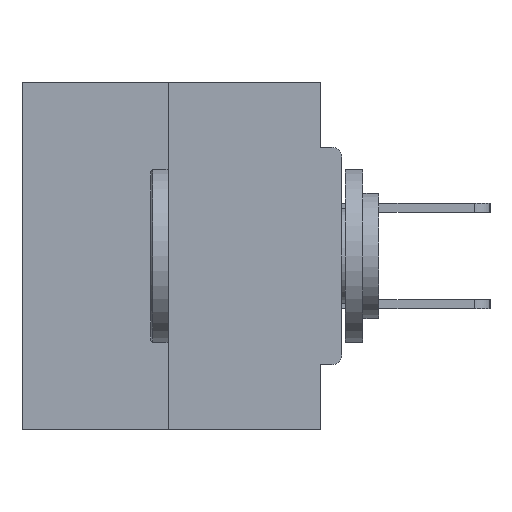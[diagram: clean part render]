
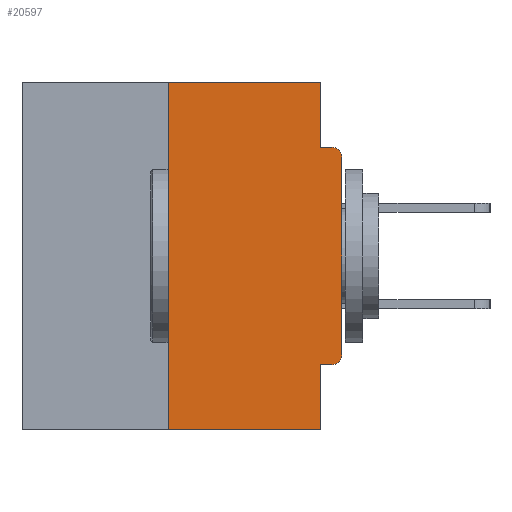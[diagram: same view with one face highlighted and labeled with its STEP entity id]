
A CAD part, left-side view. The second image highlights one B-rep face of the part: STEP entity #20597.
In plain terms, the highlighted planar face has unit normal (-1, 0, 0).
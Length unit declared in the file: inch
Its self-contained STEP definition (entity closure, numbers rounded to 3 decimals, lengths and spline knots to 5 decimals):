
#204 = LINE ( 'NONE', #33805, #28159 ) ;
#296 = ORIENTED_EDGE ( 'NONE', *, *, #18567, .F. ) ;
#996 = EDGE_CURVE ( 'NONE', #21128, #29124, #10618, .T. ) ;
#1128 = VECTOR ( 'NONE', #10268, 39.37008 ) ;
#2202 = VECTOR ( 'NONE', #10161, 39.37008 ) ;
#2663 = LINE ( 'NONE', #18475, #2202 ) ;
#3200 = EDGE_CURVE ( 'NONE', #29124, #3652, #204, .T. ) ;
#3307 = DIRECTION ( 'NONE',  ( 0., 0., -1. ) ) ;
#3652 = VERTEX_POINT ( 'NONE', #15938 ) ;
#4697 = CIRCLE ( 'NONE', #22567, 0.015 ) ;
#4855 = CARTESIAN_POINT ( 'NONE',  ( 0., 0.015, -0.4065 ) ) ;
#5638 = EDGE_CURVE ( 'NONE', #28299, #8201, #22615, .T. ) ;
#5758 = VECTOR ( 'NONE', #8541, 39.37008 ) ;
#5893 = EDGE_LOOP ( 'NONE', ( #32240, #16080, #33686, #9044, #9301, #25799, #20380, #15599, #296, #11956 ) ) ;
#5894 = CARTESIAN_POINT ( 'NONE',  ( 0., 0.25, -0.5 ) ) ;
#6037 = VECTOR ( 'NONE', #35505, 39.37008 ) ;
#6777 = PLANE ( 'NONE',  #25601 ) ;
#7136 = CARTESIAN_POINT ( 'NONE',  ( 0., 0.031, -0.5 ) ) ;
#7481 = VECTOR ( 'NONE', #20732, 39.37008 ) ;
#8165 = EDGE_CURVE ( 'NONE', #32360, #8201, #20238, .T. ) ;
#8201 = VERTEX_POINT ( 'NONE', #30403 ) ;
#8541 = DIRECTION ( 'NONE',  ( 0., -1., 0. ) ) ;
#9044 = ORIENTED_EDGE ( 'NONE', *, *, #8165, .F. ) ;
#9251 = CARTESIAN_POINT ( 'NONE',  ( 0., 0.015, -0.0935 ) ) ;
#9301 = ORIENTED_EDGE ( 'NONE', *, *, #29489, .F. ) ;
#10161 = DIRECTION ( 'NONE',  ( 0., 0., 1. ) ) ;
#10268 = DIRECTION ( 'NONE',  ( 0., 0., 1. ) ) ;
#10618 = LINE ( 'NONE', #22727, #5758 ) ;
#10646 = CARTESIAN_POINT ( 'NONE',  ( 0., 0.25, 0. ) ) ;
#10975 = CARTESIAN_POINT ( 'NONE',  ( 0., 0.031, -0.4065 ) ) ;
#11922 = AXIS2_PLACEMENT_3D ( 'NONE', #17479, #20595, #20360 ) ;
#11956 = ORIENTED_EDGE ( 'NONE', *, *, #3200, .F. ) ;
#12156 = VERTEX_POINT ( 'NONE', #12800 ) ;
#12324 = FACE_OUTER_BOUND ( 'NONE', #5893, .T. ) ;
#12800 = CARTESIAN_POINT ( 'NONE',  ( 0., 0., -0.1085 ) ) ;
#13571 = DIRECTION ( 'NONE',  ( 0., -1., 0. ) ) ;
#14453 = DIRECTION ( 'NONE',  ( -1., 0., 0. ) ) ;
#14869 = EDGE_CURVE ( 'NONE', #28299, #21128, #16214, .T. ) ;
#15599 = ORIENTED_EDGE ( 'NONE', *, *, #27118, .T. ) ;
#15611 = VERTEX_POINT ( 'NONE', #25151 ) ;
#15931 = VERTEX_POINT ( 'NONE', #4855 ) ;
#15938 = CARTESIAN_POINT ( 'NONE',  ( 0., 0.031, -0.0935 ) ) ;
#16080 = ORIENTED_EDGE ( 'NONE', *, *, #14869, .F. ) ;
#16214 = LINE ( 'NONE', #10646, #1128 ) ;
#17479 = CARTESIAN_POINT ( 'NONE',  ( 0., 0.015, -0.1085 ) ) ;
#18192 = EDGE_CURVE ( 'NONE', #15611, #12156, #2663, .T. ) ;
#18475 = CARTESIAN_POINT ( 'NONE',  ( 0., 0., 0. ) ) ;
#18567 = EDGE_CURVE ( 'NONE', #3652, #20509, #22167, .T. ) ;
#18777 = CARTESIAN_POINT ( 'NONE',  ( 0., 0.25, 0. ) ) ;
#19826 = DIRECTION ( 'NONE',  ( 0., 0., -1. ) ) ;
#20068 = DIRECTION ( 'NONE',  ( 0., 1., 0. ) ) ;
#20238 = LINE ( 'NONE', #7136, #6037 ) ;
#20360 = DIRECTION ( 'NONE',  ( 0., 0., -1. ) ) ;
#20380 = ORIENTED_EDGE ( 'NONE', *, *, #18192, .T. ) ;
#20509 = VERTEX_POINT ( 'NONE', #9251 ) ;
#20595 = DIRECTION ( 'NONE',  ( -1., 0., 0. ) ) ;
#20597 = ADVANCED_FACE ( 'NONE', ( #12324 ), #6777, .F. ) ;
#20599 = CARTESIAN_POINT ( 'NONE',  ( 0., 0.031, 0. ) ) ;
#20732 = DIRECTION ( 'NONE',  ( 0., -1., 0. ) ) ;
#21128 = VERTEX_POINT ( 'NONE', #18777 ) ;
#21889 = CARTESIAN_POINT ( 'NONE',  ( 0., 0., -0.0935 ) ) ;
#22167 = LINE ( 'NONE', #21889, #35033 ) ;
#22567 = AXIS2_PLACEMENT_3D ( 'NONE', #31527, #14453, #3307 ) ;
#22615 = LINE ( 'NONE', #23828, #7481 ) ;
#22724 = EDGE_CURVE ( 'NONE', #15931, #15611, #4697, .T. ) ;
#22727 = CARTESIAN_POINT ( 'NONE',  ( 0., 0.46, 0. ) ) ;
#23828 = CARTESIAN_POINT ( 'NONE',  ( 0., 0.46, -0.5 ) ) ;
#24426 = CIRCLE ( 'NONE', #11922, 0.015 ) ;
#24692 = VECTOR ( 'NONE', #20068, 39.37008 ) ;
#25151 = CARTESIAN_POINT ( 'NONE',  ( 0., 0., -0.3915 ) ) ;
#25601 = AXIS2_PLACEMENT_3D ( 'NONE', #29775, #35370, #26772 ) ;
#25799 = ORIENTED_EDGE ( 'NONE', *, *, #22724, .T. ) ;
#26772 = DIRECTION ( 'NONE',  ( 0., 0., -1. ) ) ;
#27118 = EDGE_CURVE ( 'NONE', #12156, #20509, #24426, .T. ) ;
#28159 = VECTOR ( 'NONE', #19826, 39.37008 ) ;
#28299 = VERTEX_POINT ( 'NONE', #5894 ) ;
#29124 = VERTEX_POINT ( 'NONE', #20599 ) ;
#29489 = EDGE_CURVE ( 'NONE', #15931, #32360, #32279, .T. ) ;
#29775 = CARTESIAN_POINT ( 'NONE',  ( 0., 0.46, 0. ) ) ;
#30403 = CARTESIAN_POINT ( 'NONE',  ( 0., 0.031, -0.5 ) ) ;
#31527 = CARTESIAN_POINT ( 'NONE',  ( 0., 0.015, -0.3915 ) ) ;
#32240 = ORIENTED_EDGE ( 'NONE', *, *, #996, .F. ) ;
#32279 = LINE ( 'NONE', #36655, #24692 ) ;
#32360 = VERTEX_POINT ( 'NONE', #10975 ) ;
#33686 = ORIENTED_EDGE ( 'NONE', *, *, #5638, .T. ) ;
#33805 = CARTESIAN_POINT ( 'NONE',  ( 0., 0.031, 0. ) ) ;
#35033 = VECTOR ( 'NONE', #13571, 39.37008 ) ;
#35370 = DIRECTION ( 'NONE',  ( 1., 0., 0. ) ) ;
#35505 = DIRECTION ( 'NONE',  ( 0., 0., -1. ) ) ;
#36655 = CARTESIAN_POINT ( 'NONE',  ( 0., 0., -0.4065 ) ) ;
